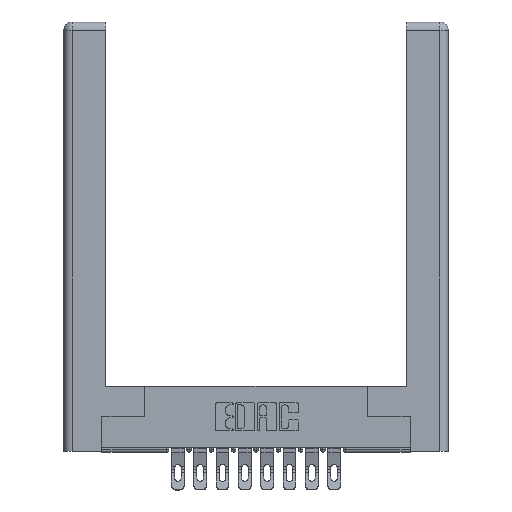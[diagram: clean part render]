
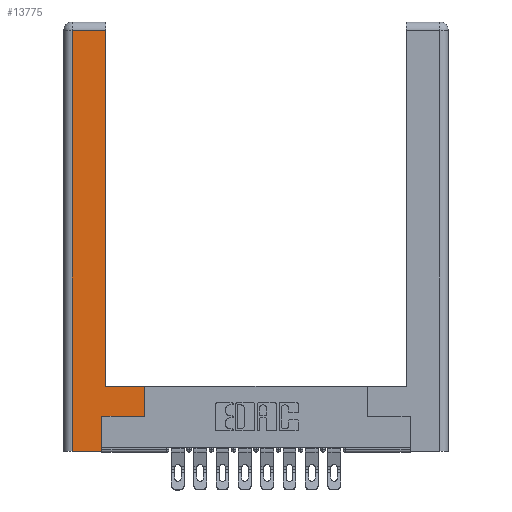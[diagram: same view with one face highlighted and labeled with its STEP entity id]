
A CAD part, top view. The second image highlights one B-rep face of the part: STEP entity #13775.
In plain terms, the highlighted planar face has unit normal (0, 0, 1).
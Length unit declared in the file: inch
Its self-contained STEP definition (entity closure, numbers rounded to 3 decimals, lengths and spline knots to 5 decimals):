
#369 = DIRECTION ( 'NONE',  ( -1., 0., 0. ) ) ;
#586 = CARTESIAN_POINT ( 'NONE',  ( 0.265, 0.245, 0. ) ) ;
#688 = EDGE_CURVE ( 'NONE', #5531, #7280, #13119, .T. ) ;
#916 = DIRECTION ( 'NONE',  ( 0., 1., 0. ) ) ;
#1187 = CARTESIAN_POINT ( 'NONE',  ( 0.565, 0.45, 0. ) ) ;
#1366 = EDGE_LOOP ( 'NONE', ( #13744, #7222, #5660, #11005, #2272, #2482, #10333, #1398 ) ) ;
#1398 = ORIENTED_EDGE ( 'NONE', *, *, #5544, .T. ) ;
#1812 = CARTESIAN_POINT ( 'NONE',  ( 0.295, 0.45, 0. ) ) ;
#2272 = ORIENTED_EDGE ( 'NONE', *, *, #2495, .T. ) ;
#2459 = EDGE_CURVE ( 'NONE', #11259, #7207, #5050, .T. ) ;
#2482 = ORIENTED_EDGE ( 'NONE', *, *, #11765, .T. ) ;
#2495 = EDGE_CURVE ( 'NONE', #15462, #3890, #8402, .T. ) ;
#2982 = CARTESIAN_POINT ( 'NONE',  ( 0.565, 0.245, 0. ) ) ;
#3015 = DIRECTION ( 'NONE',  ( 0., 1., 0. ) ) ;
#3039 = CARTESIAN_POINT ( 'NONE',  ( 0.295, 0.45, 0. ) ) ;
#3040 = VECTOR ( 'NONE', #15792, 39.37008 ) ;
#3890 = VERTEX_POINT ( 'NONE', #586 ) ;
#4111 = DIRECTION ( 'NONE',  ( 0., -1., 0. ) ) ;
#4400 = LINE ( 'NONE', #14963, #6161 ) ;
#4966 = CARTESIAN_POINT ( 'NONE',  ( 0.295, 2.94, 0. ) ) ;
#5050 = LINE ( 'NONE', #9244, #14615 ) ;
#5519 = VECTOR ( 'NONE', #916, 39.37008 ) ;
#5531 = VERTEX_POINT ( 'NONE', #2982 ) ;
#5544 = EDGE_CURVE ( 'NONE', #7280, #14127, #9698, .T. ) ;
#5570 = CARTESIAN_POINT ( 'NONE',  ( 0.265, 0., 0. ) ) ;
#5610 = VECTOR ( 'NONE', #9810, 39.37008 ) ;
#5660 = ORIENTED_EDGE ( 'NONE', *, *, #10859, .T. ) ;
#6039 = DIRECTION ( 'NONE',  ( 1., 0., 0. ) ) ;
#6161 = VECTOR ( 'NONE', #7509, 39.37008 ) ;
#6381 = LINE ( 'NONE', #15958, #5610 ) ;
#6551 = CARTESIAN_POINT ( 'NONE',  ( 0., 0., 0. ) ) ;
#7104 = CARTESIAN_POINT ( 'NONE',  ( 0.0615, 2.94, 0. ) ) ;
#7207 = VERTEX_POINT ( 'NONE', #7104 ) ;
#7222 = ORIENTED_EDGE ( 'NONE', *, *, #2459, .T. ) ;
#7280 = VERTEX_POINT ( 'NONE', #1187 ) ;
#7509 = DIRECTION ( 'NONE',  ( 0., 1., 0. ) ) ;
#8229 = DIRECTION ( 'NONE',  ( -1., 0., 0. ) ) ;
#8349 = CARTESIAN_POINT ( 'NONE',  ( 0.0615, 0., 0. ) ) ;
#8402 = LINE ( 'NONE', #10505, #9772 ) ;
#8526 = CARTESIAN_POINT ( 'NONE',  ( 0.565, 0.45, 0. ) ) ;
#9126 = VERTEX_POINT ( 'NONE', #8349 ) ;
#9244 = CARTESIAN_POINT ( 'NONE',  ( 0.0615, 2.94, 0. ) ) ;
#9595 = VECTOR ( 'NONE', #6039, 39.37008 ) ;
#9698 = LINE ( 'NONE', #3039, #3040 ) ;
#9772 = VECTOR ( 'NONE', #3015, 39.37008 ) ;
#9810 = DIRECTION ( 'NONE',  ( 1., 0., 0. ) ) ;
#10293 = AXIS2_PLACEMENT_3D ( 'NONE', #6551, #13248, #8229 ) ;
#10333 = ORIENTED_EDGE ( 'NONE', *, *, #688, .T. ) ;
#10505 = CARTESIAN_POINT ( 'NONE',  ( 0.265, 0.245, 0. ) ) ;
#10859 = EDGE_CURVE ( 'NONE', #7207, #9126, #13832, .T. ) ;
#11005 = ORIENTED_EDGE ( 'NONE', *, *, #13712, .T. ) ;
#11259 = VERTEX_POINT ( 'NONE', #4966 ) ;
#11765 = EDGE_CURVE ( 'NONE', #3890, #5531, #6381, .T. ) ;
#11824 = CARTESIAN_POINT ( 'NONE',  ( 0.0615, 0., 0. ) ) ;
#11913 = VECTOR ( 'NONE', #4111, 39.37008 ) ;
#12316 = FACE_OUTER_BOUND ( 'NONE', #1366, .T. ) ;
#12684 = PLANE ( 'NONE',  #10293 ) ;
#13119 = LINE ( 'NONE', #8526, #5519 ) ;
#13248 = DIRECTION ( 'NONE',  ( 0., 0., -1. ) ) ;
#13346 = CARTESIAN_POINT ( 'NONE',  ( 0.265, 0., 0. ) ) ;
#13477 = LINE ( 'NONE', #13346, #9595 ) ;
#13712 = EDGE_CURVE ( 'NONE', #9126, #15462, #13477, .T. ) ;
#13744 = ORIENTED_EDGE ( 'NONE', *, *, #15805, .T. ) ;
#13775 = ADVANCED_FACE ( 'NONE', ( #12316 ), #12684, .F. ) ;
#13832 = LINE ( 'NONE', #11824, #11913 ) ;
#14127 = VERTEX_POINT ( 'NONE', #1812 ) ;
#14615 = VECTOR ( 'NONE', #369, 39.37008 ) ;
#14963 = CARTESIAN_POINT ( 'NONE',  ( 0.295, 3., 0. ) ) ;
#15462 = VERTEX_POINT ( 'NONE', #5570 ) ;
#15792 = DIRECTION ( 'NONE',  ( -1., 0., 0. ) ) ;
#15805 = EDGE_CURVE ( 'NONE', #14127, #11259, #4400, .T. ) ;
#15958 = CARTESIAN_POINT ( 'NONE',  ( 0.565, 0.245, 0. ) ) ;
